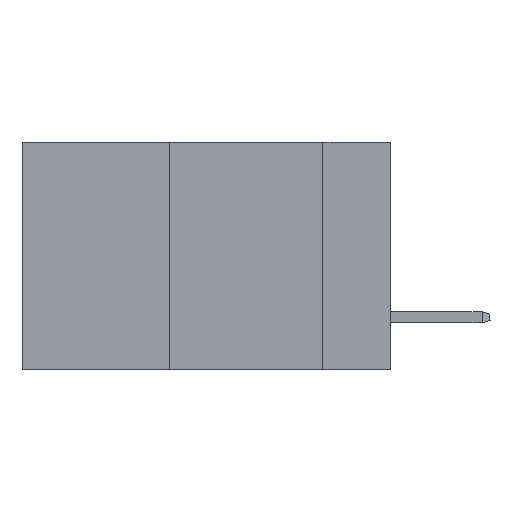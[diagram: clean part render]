
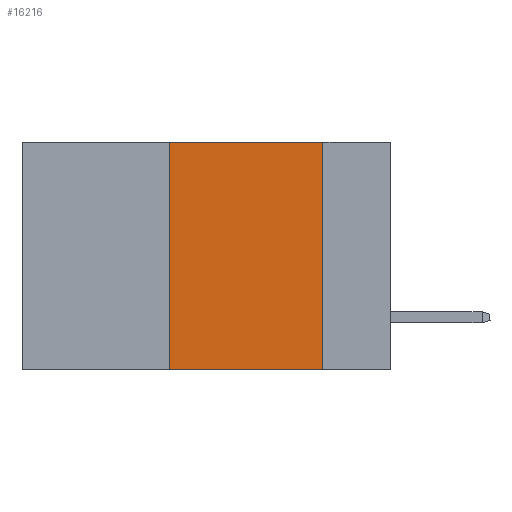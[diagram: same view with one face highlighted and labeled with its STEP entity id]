
A CAD part, left-side view. The second image highlights one B-rep face of the part: STEP entity #16216.
In plain terms, the highlighted planar face has unit normal (-1, 0, 0).
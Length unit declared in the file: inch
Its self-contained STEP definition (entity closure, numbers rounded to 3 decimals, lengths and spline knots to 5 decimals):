
#44 = VERTEX_POINT ( 'NONE', #5825 ) ;
#1038 = ORIENTED_EDGE ( 'NONE', *, *, #11957, .T. ) ;
#1771 = CARTESIAN_POINT ( 'NONE',  ( 0., 0.11, 0. ) ) ;
#2640 = DIRECTION ( 'NONE',  ( 0., 0., 1. ) ) ;
#2987 = CARTESIAN_POINT ( 'NONE',  ( 0., 0.6, -0.37 ) ) ;
#4106 = VECTOR ( 'NONE', #15663, 39.37008 ) ;
#4137 = EDGE_LOOP ( 'NONE', ( #14616, #16826, #4448, #1038 ) ) ;
#4448 = ORIENTED_EDGE ( 'NONE', *, *, #7649, .F. ) ;
#4507 = VECTOR ( 'NONE', #2640, 39.37008 ) ;
#4988 = DIRECTION ( 'NONE',  ( 0., 0., -1. ) ) ;
#5505 = VERTEX_POINT ( 'NONE', #7068 ) ;
#5825 = CARTESIAN_POINT ( 'NONE',  ( 0., 0.11, -0.37 ) ) ;
#6183 = LINE ( 'NONE', #7971, #7662 ) ;
#7068 = CARTESIAN_POINT ( 'NONE',  ( 0., 0.36, 0. ) ) ;
#7649 = EDGE_CURVE ( 'NONE', #19698, #5505, #8506, .T. ) ;
#7662 = VECTOR ( 'NONE', #12524, 39.37008 ) ;
#7971 = CARTESIAN_POINT ( 'NONE',  ( 0., 0.6, 0. ) ) ;
#8169 = FACE_OUTER_BOUND ( 'NONE', #4137, .T. ) ;
#8506 = LINE ( 'NONE', #16728, #4507 ) ;
#9792 = PLANE ( 'NONE',  #13605 ) ;
#9982 = LINE ( 'NONE', #1771, #11486 ) ;
#10895 = EDGE_CURVE ( 'NONE', #5505, #17371, #6183, .T. ) ;
#11486 = VECTOR ( 'NONE', #4988, 39.37008 ) ;
#11534 = DIRECTION ( 'NONE',  ( 0., 0., -1. ) ) ;
#11807 = CARTESIAN_POINT ( 'NONE',  ( 0., 0.36, -0.37 ) ) ;
#11957 = EDGE_CURVE ( 'NONE', #19698, #44, #15090, .T. ) ;
#12524 = DIRECTION ( 'NONE',  ( 0., -1., 0. ) ) ;
#13605 = AXIS2_PLACEMENT_3D ( 'NONE', #16486, #17727, #11534 ) ;
#14616 = ORIENTED_EDGE ( 'NONE', *, *, #18041, .F. ) ;
#15090 = LINE ( 'NONE', #2987, #4106 ) ;
#15663 = DIRECTION ( 'NONE',  ( 0., -1., 0. ) ) ;
#16216 = ADVANCED_FACE ( 'NONE', ( #8169 ), #9792, .F. ) ;
#16486 = CARTESIAN_POINT ( 'NONE',  ( 0., 0.6, 0. ) ) ;
#16728 = CARTESIAN_POINT ( 'NONE',  ( 0., 0.36, 0. ) ) ;
#16826 = ORIENTED_EDGE ( 'NONE', *, *, #10895, .F. ) ;
#17371 = VERTEX_POINT ( 'NONE', #17468 ) ;
#17468 = CARTESIAN_POINT ( 'NONE',  ( 0., 0.11, 0. ) ) ;
#17727 = DIRECTION ( 'NONE',  ( 1., 0., 0. ) ) ;
#18041 = EDGE_CURVE ( 'NONE', #17371, #44, #9982, .T. ) ;
#19698 = VERTEX_POINT ( 'NONE', #11807 ) ;
